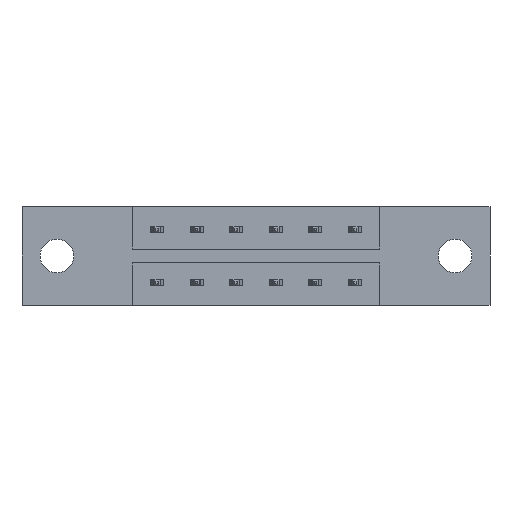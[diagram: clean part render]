
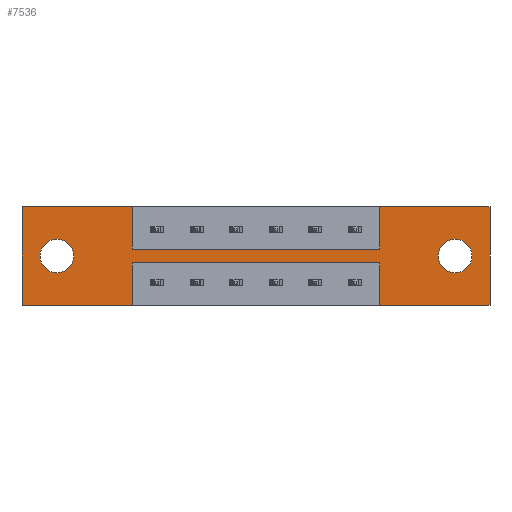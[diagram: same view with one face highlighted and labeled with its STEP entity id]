
A CAD part, front view. The second image highlights one B-rep face of the part: STEP entity #7536.
In plain terms, the highlighted planar face has unit normal (0, -1, 0).
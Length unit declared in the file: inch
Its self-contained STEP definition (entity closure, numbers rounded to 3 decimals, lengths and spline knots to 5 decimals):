
#120 = ORIENTED_EDGE ( 'NONE', *, *, #585, .F. ) ;
#130 = FACE_BOUND ( 'NONE', #1438, .T. ) ;
#132 = ORIENTED_EDGE ( 'NONE', *, *, #800, .T. ) ;
#162 = VERTEX_POINT ( 'NONE', #6181 ) ;
#223 = VERTEX_POINT ( 'NONE', #2220 ) ;
#232 = DIRECTION ( 'NONE',  ( 0., 0., -1. ) ) ;
#275 = CIRCLE ( 'NONE', #4663, 0.064 ) ;
#339 = FACE_BOUND ( 'NONE', #5058, .T. ) ;
#357 = DIRECTION ( 'NONE',  ( 0., 0., -1. ) ) ;
#398 = CARTESIAN_POINT ( 'NONE',  ( 0.1325, 0., -0.1875 ) ) ;
#452 = VERTEX_POINT ( 'NONE', #4449 ) ;
#502 = LINE ( 'NONE', #996, #2560 ) ;
#523 = VERTEX_POINT ( 'NONE', #4000 ) ;
#554 = CIRCLE ( 'NONE', #1613, 0.064 ) ;
#585 = EDGE_CURVE ( 'NONE', #7246, #6377, #3116, .T. ) ;
#725 = VECTOR ( 'NONE', #7311, 39.37008 ) ;
#728 = CARTESIAN_POINT ( 'NONE',  ( 0.4175, 0., -0.214 ) ) ;
#800 = EDGE_CURVE ( 'NONE', #6076, #4482, #4652, .T. ) ;
#914 = DIRECTION ( 'NONE',  ( 0., 0., -1. ) ) ;
#996 = CARTESIAN_POINT ( 'NONE',  ( 0., 0., -0.375 ) ) ;
#1087 = DIRECTION ( 'NONE',  ( 0., 1., 0. ) ) ;
#1139 = EDGE_LOOP ( 'NONE', ( #7952, #5030, #7709, #8137, #120, #7840, #1145, #6932, #6984, #4374, #3872, #4968 ) ) ;
#1145 = ORIENTED_EDGE ( 'NONE', *, *, #6952, .F. ) ;
#1438 = EDGE_LOOP ( 'NONE', ( #3258, #2157 ) ) ;
#1460 = DIRECTION ( 'NONE',  ( 0., -1., 0. ) ) ;
#1501 = EDGE_CURVE ( 'NONE', #1540, #3946, #4530, .T. ) ;
#1513 = LINE ( 'NONE', #3414, #8341 ) ;
#1540 = VERTEX_POINT ( 'NONE', #2522 ) ;
#1613 = AXIS2_PLACEMENT_3D ( 'NONE', #5645, #2978, #357 ) ;
#1631 = ORIENTED_EDGE ( 'NONE', *, *, #5419, .T. ) ;
#1684 = EDGE_CURVE ( 'NONE', #3946, #162, #4843, .T. ) ;
#2005 = CARTESIAN_POINT ( 'NONE',  ( 0.4175, 0., -0.161 ) ) ;
#2157 = ORIENTED_EDGE ( 'NONE', *, *, #7194, .T. ) ;
#2205 = LINE ( 'NONE', #2005, #7683 ) ;
#2219 = VERTEX_POINT ( 'NONE', #6461 ) ;
#2220 = CARTESIAN_POINT ( 'NONE',  ( 1.6425, 0., -0.2515 ) ) ;
#2418 = CARTESIAN_POINT ( 'NONE',  ( 1.3575, 0., -0.214 ) ) ;
#2509 = CIRCLE ( 'NONE', #6674, 0.064 ) ;
#2522 = CARTESIAN_POINT ( 'NONE',  ( 1.3575, 0., -0.375 ) ) ;
#2560 = VECTOR ( 'NONE', #5603, 39.37008 ) ;
#2622 = CARTESIAN_POINT ( 'NONE',  ( 0.1325, 0., -0.1235 ) ) ;
#2649 = CARTESIAN_POINT ( 'NONE',  ( 0.4175, 0., -0.161 ) ) ;
#2657 = CARTESIAN_POINT ( 'NONE',  ( 1.3575, 0., -0.161 ) ) ;
#2764 = DIRECTION ( 'NONE',  ( 0., 0., -1. ) ) ;
#2978 = DIRECTION ( 'NONE',  ( 0., 1., 0. ) ) ;
#3116 = LINE ( 'NONE', #2657, #7771 ) ;
#3253 = VERTEX_POINT ( 'NONE', #6355 ) ;
#3258 = ORIENTED_EDGE ( 'NONE', *, *, #7201, .T. ) ;
#3270 = CARTESIAN_POINT ( 'NONE',  ( 0., 0., 0. ) ) ;
#3323 = VERTEX_POINT ( 'NONE', #4470 ) ;
#3338 = VECTOR ( 'NONE', #6086, 39.37008 ) ;
#3372 = DIRECTION ( 'NONE',  ( 0., 0., 1. ) ) ;
#3411 = PLANE ( 'NONE',  #8387 ) ;
#3414 = CARTESIAN_POINT ( 'NONE',  ( 0., 0., 0. ) ) ;
#3420 = DIRECTION ( 'NONE',  ( 1., 0., 0. ) ) ;
#3424 = LINE ( 'NONE', #8115, #8469 ) ;
#3470 = EDGE_CURVE ( 'NONE', #6377, #2219, #1513, .T. ) ;
#3496 = DIRECTION ( 'NONE',  ( 0., 0., -1. ) ) ;
#3754 = EDGE_CURVE ( 'NONE', #523, #452, #502, .T. ) ;
#3762 = DIRECTION ( 'NONE',  ( 0., 0., 1. ) ) ;
#3872 = ORIENTED_EDGE ( 'NONE', *, *, #6511, .F. ) ;
#3905 = DIRECTION ( 'NONE',  ( 0., 0., 1. ) ) ;
#3946 = VERTEX_POINT ( 'NONE', #2418 ) ;
#3983 = VECTOR ( 'NONE', #3496, 39.37008 ) ;
#4000 = CARTESIAN_POINT ( 'NONE',  ( 0.4175, 0., -0.375 ) ) ;
#4054 = LINE ( 'NONE', #6800, #3338 ) ;
#4082 = DIRECTION ( 'NONE',  ( 0., 1., 0. ) ) ;
#4284 = LINE ( 'NONE', #6797, #3983 ) ;
#4334 = CARTESIAN_POINT ( 'NONE',  ( 1.3575, 0., -0.161 ) ) ;
#4374 = ORIENTED_EDGE ( 'NONE', *, *, #3754, .F. ) ;
#4449 = CARTESIAN_POINT ( 'NONE',  ( 0., 0., -0.375 ) ) ;
#4470 = CARTESIAN_POINT ( 'NONE',  ( 1.6425, 0., -0.1235 ) ) ;
#4482 = VERTEX_POINT ( 'NONE', #2622 ) ;
#4530 = LINE ( 'NONE', #4564, #7029 ) ;
#4564 = CARTESIAN_POINT ( 'NONE',  ( 1.3575, 0., -0.214 ) ) ;
#4608 = DIRECTION ( 'NONE',  ( 1., 0., 0. ) ) ;
#4652 = CIRCLE ( 'NONE', #8035, 0.064 ) ;
#4663 = AXIS2_PLACEMENT_3D ( 'NONE', #7423, #4082, #6082 ) ;
#4754 = VECTOR ( 'NONE', #3420, 39.37008 ) ;
#4843 = LINE ( 'NONE', #728, #725 ) ;
#4855 = CARTESIAN_POINT ( 'NONE',  ( 1.6425, 0., -0.1875 ) ) ;
#4968 = ORIENTED_EDGE ( 'NONE', *, *, #1684, .F. ) ;
#5030 = ORIENTED_EDGE ( 'NONE', *, *, #7714, .F. ) ;
#5058 = EDGE_LOOP ( 'NONE', ( #1631, #132 ) ) ;
#5060 = VERTEX_POINT ( 'NONE', #6207 ) ;
#5285 = CARTESIAN_POINT ( 'NONE',  ( 0.4175, 0., -0.161 ) ) ;
#5318 = VERTEX_POINT ( 'NONE', #2649 ) ;
#5355 = EDGE_CURVE ( 'NONE', #6236, #5060, #8417, .T. ) ;
#5419 = EDGE_CURVE ( 'NONE', #4482, #6076, #275, .T. ) ;
#5563 = DIRECTION ( 'NONE',  ( 0., 1., 0. ) ) ;
#5603 = DIRECTION ( 'NONE',  ( -1., 0., 0. ) ) ;
#5645 = CARTESIAN_POINT ( 'NONE',  ( 1.6425, 0., -0.1875 ) ) ;
#5890 = FACE_OUTER_BOUND ( 'NONE', #1139, .T. ) ;
#5928 = CARTESIAN_POINT ( 'NONE',  ( 0., 0., -0.375 ) ) ;
#6076 = VERTEX_POINT ( 'NONE', #6357 ) ;
#6082 = DIRECTION ( 'NONE',  ( 0., 0., 1. ) ) ;
#6086 = DIRECTION ( 'NONE',  ( -1., 0., 0. ) ) ;
#6181 = CARTESIAN_POINT ( 'NONE',  ( 0.4175, 0., -0.214 ) ) ;
#6207 = CARTESIAN_POINT ( 'NONE',  ( 0.4175, 0., 0. ) ) ;
#6236 = VERTEX_POINT ( 'NONE', #6470 ) ;
#6355 = CARTESIAN_POINT ( 'NONE',  ( 1.775, 0., -0.375 ) ) ;
#6357 = CARTESIAN_POINT ( 'NONE',  ( 0.1325, 0., -0.2515 ) ) ;
#6377 = VERTEX_POINT ( 'NONE', #7306 ) ;
#6461 = CARTESIAN_POINT ( 'NONE',  ( 1.775, 0., 0. ) ) ;
#6470 = CARTESIAN_POINT ( 'NONE',  ( 0., 0., 0. ) ) ;
#6511 = EDGE_CURVE ( 'NONE', #162, #523, #4284, .T. ) ;
#6516 = LINE ( 'NONE', #5285, #4754 ) ;
#6674 = AXIS2_PLACEMENT_3D ( 'NONE', #4855, #5563, #914 ) ;
#6797 = CARTESIAN_POINT ( 'NONE',  ( 0.4175, 0., -0.214 ) ) ;
#6800 = CARTESIAN_POINT ( 'NONE',  ( 0., 0., -0.375 ) ) ;
#6932 = ORIENTED_EDGE ( 'NONE', *, *, #5355, .F. ) ;
#6952 = EDGE_CURVE ( 'NONE', #5060, #5318, #2205, .T. ) ;
#6984 = ORIENTED_EDGE ( 'NONE', *, *, #8030, .F. ) ;
#7029 = VECTOR ( 'NONE', #8404, 39.37008 ) ;
#7194 = EDGE_CURVE ( 'NONE', #223, #3323, #2509, .T. ) ;
#7201 = EDGE_CURVE ( 'NONE', #3323, #223, #554, .T. ) ;
#7246 = VERTEX_POINT ( 'NONE', #4334 ) ;
#7306 = CARTESIAN_POINT ( 'NONE',  ( 1.3575, 0., 0. ) ) ;
#7311 = DIRECTION ( 'NONE',  ( -1., 0., 0. ) ) ;
#7423 = CARTESIAN_POINT ( 'NONE',  ( 0.1325, 0., -0.1875 ) ) ;
#7458 = VECTOR ( 'NONE', #3905, 39.37008 ) ;
#7536 = ADVANCED_FACE ( 'NONE', ( #130, #339, #5890 ), #3411, .T. ) ;
#7683 = VECTOR ( 'NONE', #232, 39.37008 ) ;
#7709 = ORIENTED_EDGE ( 'NONE', *, *, #8419, .F. ) ;
#7714 = EDGE_CURVE ( 'NONE', #3253, #1540, #4054, .T. ) ;
#7771 = VECTOR ( 'NONE', #3372, 39.37008 ) ;
#7827 = DIRECTION ( 'NONE',  ( 1., 0., 0. ) ) ;
#7830 = CARTESIAN_POINT ( 'NONE',  ( 0., 0., 0. ) ) ;
#7840 = ORIENTED_EDGE ( 'NONE', *, *, #8211, .F. ) ;
#7864 = LINE ( 'NONE', #7830, #7458 ) ;
#7952 = ORIENTED_EDGE ( 'NONE', *, *, #1501, .F. ) ;
#8030 = EDGE_CURVE ( 'NONE', #452, #6236, #7864, .T. ) ;
#8035 = AXIS2_PLACEMENT_3D ( 'NONE', #398, #1087, #3762 ) ;
#8115 = CARTESIAN_POINT ( 'NONE',  ( 1.775, 0., 0. ) ) ;
#8137 = ORIENTED_EDGE ( 'NONE', *, *, #3470, .F. ) ;
#8168 = DIRECTION ( 'NONE',  ( 0., 0., -1. ) ) ;
#8211 = EDGE_CURVE ( 'NONE', #5318, #7246, #6516, .T. ) ;
#8326 = VECTOR ( 'NONE', #7827, 39.37008 ) ;
#8341 = VECTOR ( 'NONE', #4608, 39.37008 ) ;
#8387 = AXIS2_PLACEMENT_3D ( 'NONE', #5928, #1460, #2764 ) ;
#8404 = DIRECTION ( 'NONE',  ( 0., 0., 1. ) ) ;
#8417 = LINE ( 'NONE', #3270, #8326 ) ;
#8419 = EDGE_CURVE ( 'NONE', #2219, #3253, #3424, .T. ) ;
#8469 = VECTOR ( 'NONE', #8168, 39.37008 ) ;
